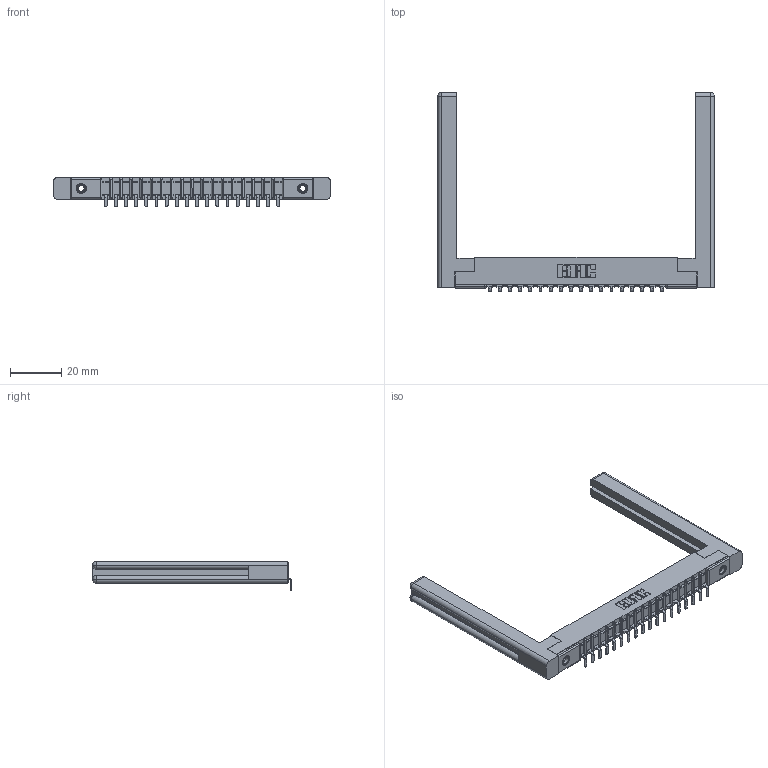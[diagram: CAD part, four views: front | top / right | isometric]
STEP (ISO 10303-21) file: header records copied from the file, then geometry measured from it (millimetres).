
FILE_DESCRIPTION (( 'STEP AP203' ), '1' );
FILE_NAME ('357-018-453-158.STEP', '2020-10-01T00:46:09', ( '' ), ( '' ), 'SwSTEP 2.0', 'SolidWorks 2020', '' );
FILE_SCHEMA (( 'CONFIG_CONTROL_DESIGN' ));
Length unit declared in the file: inch
Products named in the file (5): 307-220-058; 307 Part_.156 Dia Mounting Holes; 345-250-001_345-250-001-102; 307-290-002_553; 357-018-453-158
Assembly tree (23 placements, depth 2):
  357-018-453-158
    307 Part_.156 Dia Mounting Holes
    307-290-002_553  x18
    307-220-058  x2
    345-250-001_345-250-001-102  x2
Bounding box: 107.95 x 77.64 x 11.51 mm (x, y, z)
Volume: 14802.8 mm3; surface area: 17765.6 mm2
Topology: 23 solids, 23 shells, 1683 faces, 5069 edges, 3314 vertices
Faces by surface type: plane 1000, cylinder 621, sphere 38, torus 12, cone 12
Entity records: 21877 total; most frequent: CARTESIAN_POINT 3695, ORIENTED_EDGE 3624, DIRECTION 3562, EDGE_CURVE 1812, VECTOR 1372, LINE 1372, VERTEX_POINT 1174, AXIS2_PLACEMENT_3D 1095
